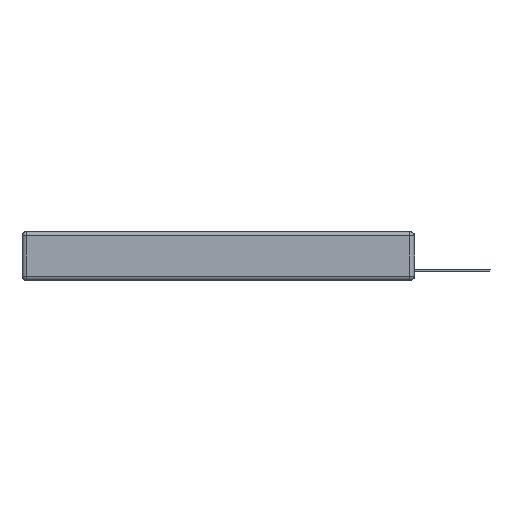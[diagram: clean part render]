
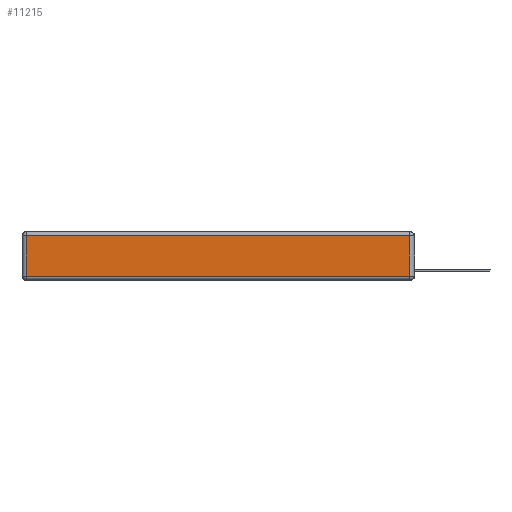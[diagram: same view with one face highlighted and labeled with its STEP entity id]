
A CAD part, left-side view. The second image highlights one B-rep face of the part: STEP entity #11215.
In plain terms, the highlighted planar face has unit normal (-1, 0, 0).
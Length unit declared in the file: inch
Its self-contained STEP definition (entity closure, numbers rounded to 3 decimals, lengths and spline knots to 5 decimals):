
#494 = LINE ( 'NONE', #2292, #24771 ) ;
#617 = EDGE_CURVE ( 'NONE', #4739, #12071, #6700, .T. ) ;
#1338 = CARTESIAN_POINT ( 'NONE',  ( 0., 0., -0.343 ) ) ;
#1465 = DIRECTION ( 'NONE',  ( -1., 0., 0. ) ) ;
#1954 = CARTESIAN_POINT ( 'NONE',  ( 0., 0.03, -0.03 ) ) ;
#2292 = CARTESIAN_POINT ( 'NONE',  ( 0., 2.72, -0.343 ) ) ;
#3340 = CARTESIAN_POINT ( 'NONE',  ( 0., 2.72, -0.03 ) ) ;
#3696 = VECTOR ( 'NONE', #10038, 39.37008 ) ;
#4739 = VERTEX_POINT ( 'NONE', #1954 ) ;
#5782 = VECTOR ( 'NONE', #18337, 39.37008 ) ;
#6182 = EDGE_LOOP ( 'NONE', ( #9927, #19577, #10990, #13686 ) ) ;
#6414 = DIRECTION ( 'NONE',  ( 0., 0., -1. ) ) ;
#6582 = CARTESIAN_POINT ( 'NONE',  ( 0., 2.72, -0.313 ) ) ;
#6700 = LINE ( 'NONE', #10467, #5782 ) ;
#7857 = CARTESIAN_POINT ( 'NONE',  ( 0., 0., -0.313 ) ) ;
#8741 = LINE ( 'NONE', #7857, #3696 ) ;
#9927 = ORIENTED_EDGE ( 'NONE', *, *, #14485, .T. ) ;
#10038 = DIRECTION ( 'NONE',  ( 0., -1., 0. ) ) ;
#10467 = CARTESIAN_POINT ( 'NONE',  ( 0., 2.75, -0.03 ) ) ;
#10990 = ORIENTED_EDGE ( 'NONE', *, *, #617, .T. ) ;
#11215 = ADVANCED_FACE ( 'NONE', ( #21115 ), #13343, .T. ) ;
#11913 = VERTEX_POINT ( 'NONE', #6582 ) ;
#12071 = VERTEX_POINT ( 'NONE', #3340 ) ;
#12886 = AXIS2_PLACEMENT_3D ( 'NONE', #1338, #1465, #21242 ) ;
#13138 = CARTESIAN_POINT ( 'NONE',  ( 0., 0.03, -0.313 ) ) ;
#13343 = PLANE ( 'NONE',  #12886 ) ;
#13598 = VERTEX_POINT ( 'NONE', #13138 ) ;
#13686 = ORIENTED_EDGE ( 'NONE', *, *, #14589, .T. ) ;
#13969 = VECTOR ( 'NONE', #14534, 39.37008 ) ;
#14485 = EDGE_CURVE ( 'NONE', #11913, #13598, #8741, .T. ) ;
#14534 = DIRECTION ( 'NONE',  ( 0., 0., 1. ) ) ;
#14589 = EDGE_CURVE ( 'NONE', #12071, #11913, #494, .T. ) ;
#16600 = CARTESIAN_POINT ( 'NONE',  ( 0., 0.03, -0.343 ) ) ;
#18337 = DIRECTION ( 'NONE',  ( 0., 1., 0. ) ) ;
#19183 = EDGE_CURVE ( 'NONE', #13598, #4739, #24117, .T. ) ;
#19577 = ORIENTED_EDGE ( 'NONE', *, *, #19183, .T. ) ;
#21115 = FACE_OUTER_BOUND ( 'NONE', #6182, .T. ) ;
#21242 = DIRECTION ( 'NONE',  ( 0., 0., 1. ) ) ;
#24117 = LINE ( 'NONE', #16600, #13969 ) ;
#24771 = VECTOR ( 'NONE', #6414, 39.37008 ) ;
